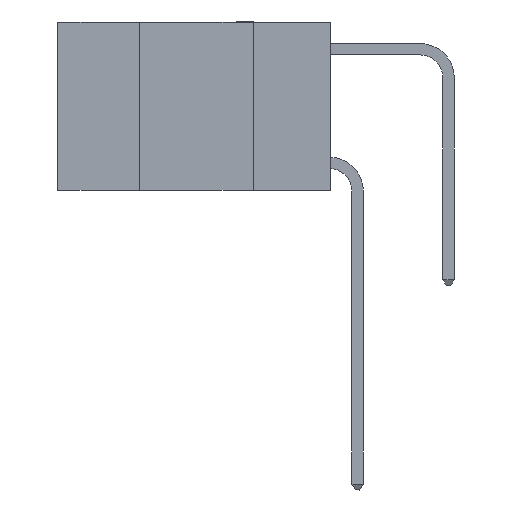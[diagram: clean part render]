
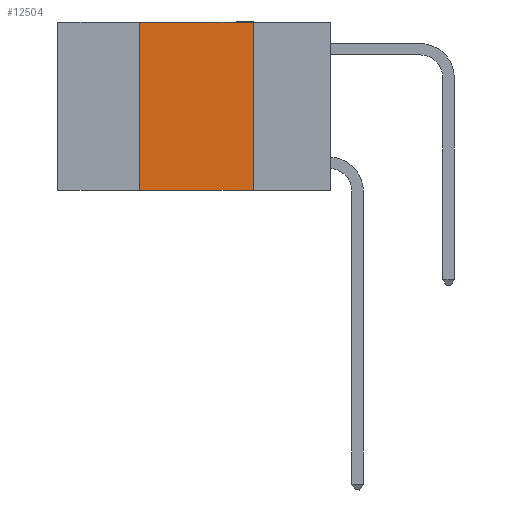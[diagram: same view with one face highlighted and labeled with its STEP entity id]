
A CAD part, left-side view. The second image highlights one B-rep face of the part: STEP entity #12504.
In plain terms, the highlighted planar face has unit normal (-1, 0, 0).
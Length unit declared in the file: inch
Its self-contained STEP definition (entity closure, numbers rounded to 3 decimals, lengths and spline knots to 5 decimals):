
#118 = CARTESIAN_POINT ( 'NONE',  ( 0., 0.42, -0.37 ) ) ;
#167 = DIRECTION ( 'NONE',  ( 0., 0., 1. ) ) ;
#800 = EDGE_CURVE ( 'NONE', #6520, #9366, #942, .T. ) ;
#942 = LINE ( 'NONE', #6141, #2994 ) ;
#1112 = ORIENTED_EDGE ( 'NONE', *, *, #16526, .T. ) ;
#2994 = VECTOR ( 'NONE', #11901, 39.37008 ) ;
#4249 = ORIENTED_EDGE ( 'NONE', *, *, #17479, .F. ) ;
#4426 = PLANE ( 'NONE',  #18186 ) ;
#4646 = CARTESIAN_POINT ( 'NONE',  ( 0., 0.42, 0. ) ) ;
#4747 = LINE ( 'NONE', #16938, #15066 ) ;
#5103 = FACE_OUTER_BOUND ( 'NONE', #17050, .T. ) ;
#5545 = CARTESIAN_POINT ( 'NONE',  ( 0., 0.17, 0. ) ) ;
#5871 = VECTOR ( 'NONE', #167, 39.37008 ) ;
#6141 = CARTESIAN_POINT ( 'NONE',  ( 0., 0.6, 0. ) ) ;
#6322 = LINE ( 'NONE', #4646, #5871 ) ;
#6520 = VERTEX_POINT ( 'NONE', #17071 ) ;
#7792 = CARTESIAN_POINT ( 'NONE',  ( 0., 0.6, 0. ) ) ;
#8596 = ORIENTED_EDGE ( 'NONE', *, *, #17403, .F. ) ;
#9366 = VERTEX_POINT ( 'NONE', #5545 ) ;
#10580 = VERTEX_POINT ( 'NONE', #16889 ) ;
#11007 = DIRECTION ( 'NONE',  ( 0., -1., 0. ) ) ;
#11573 = DIRECTION ( 'NONE',  ( 1., 0., 0. ) ) ;
#11901 = DIRECTION ( 'NONE',  ( 0., -1., 0. ) ) ;
#12504 = ADVANCED_FACE ( 'NONE', ( #5103 ), #4426, .F. ) ;
#15066 = VECTOR ( 'NONE', #11007, 39.37008 ) ;
#15644 = ORIENTED_EDGE ( 'NONE', *, *, #800, .F. ) ;
#15997 = DIRECTION ( 'NONE',  ( 0., 0., -1. ) ) ;
#16064 = CARTESIAN_POINT ( 'NONE',  ( 0., 0.17, 0. ) ) ;
#16419 = LINE ( 'NONE', #16064, #16880 ) ;
#16526 = EDGE_CURVE ( 'NONE', #18391, #10580, #4747, .T. ) ;
#16880 = VECTOR ( 'NONE', #15997, 39.37008 ) ;
#16889 = CARTESIAN_POINT ( 'NONE',  ( 0., 0.17, -0.37 ) ) ;
#16938 = CARTESIAN_POINT ( 'NONE',  ( 0., 0.6, -0.37 ) ) ;
#17050 = EDGE_LOOP ( 'NONE', ( #4249, #15644, #8596, #1112 ) ) ;
#17071 = CARTESIAN_POINT ( 'NONE',  ( 0., 0.42, 0. ) ) ;
#17403 = EDGE_CURVE ( 'NONE', #18391, #6520, #6322, .T. ) ;
#17479 = EDGE_CURVE ( 'NONE', #9366, #10580, #16419, .T. ) ;
#17736 = DIRECTION ( 'NONE',  ( 0., 0., -1. ) ) ;
#18186 = AXIS2_PLACEMENT_3D ( 'NONE', #7792, #11573, #17736 ) ;
#18391 = VERTEX_POINT ( 'NONE', #118 ) ;
